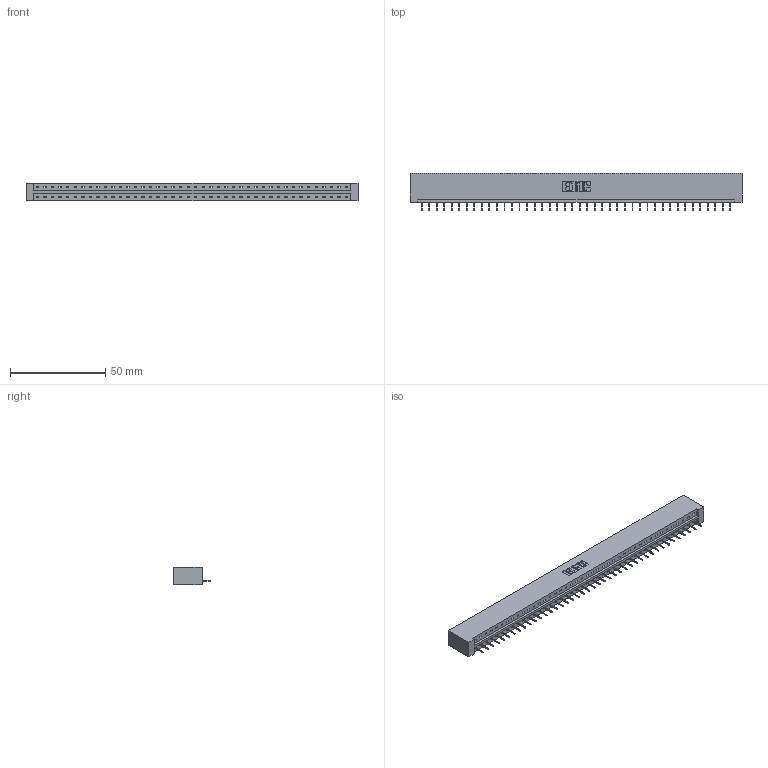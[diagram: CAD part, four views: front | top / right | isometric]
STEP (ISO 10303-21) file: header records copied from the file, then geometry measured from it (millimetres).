
FILE_DESCRIPTION (( 'STEP AP203' ), '1' );
FILE_NAME ('333-042-524-101.STEP', '2018-08-03T18:39:31', ( '' ), ( '' ), 'SwSTEP 2.0', 'SolidWorks 2016', '' );
FILE_SCHEMA (( 'CONFIG_CONTROL_DESIGN' ));
Length unit declared in the file: inch
Products named in the file (3): 333 Part_Lugless; 345-292-001_345-293-124; 333-042-524-101
Assembly tree (43 placements, depth 2):
  333-042-524-101
    333 Part_Lugless
    345-292-001_345-293-124  x42
Bounding box: 174.68 x 19.69 x 9.4 mm (x, y, z)
Volume: 18024.2 mm3; surface area: 18888.2 mm2
Topology: 43 solids, 43 shells, 2710 faces, 7847 edges, 5062 vertices
Faces by surface type: plane 2082, cylinder 628
Entity records: 25473 total; most frequent: CARTESIAN_POINT 4400, ORIENTED_EDGE 4378, DIRECTION 3705, EDGE_CURVE 2189, VECTOR 2073, LINE 2073, VERTEX_POINT 1454, AXIS2_PLACEMENT_3D 816
